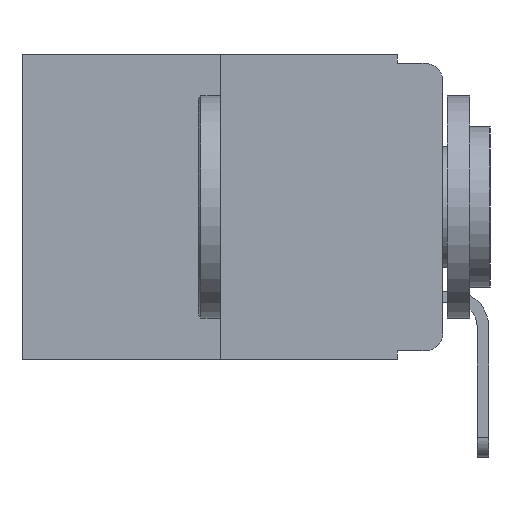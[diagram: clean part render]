
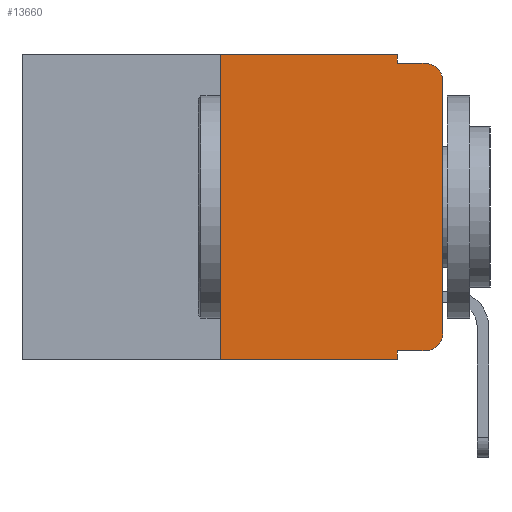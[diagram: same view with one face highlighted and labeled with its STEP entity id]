
A CAD part, left-side view. The second image highlights one B-rep face of the part: STEP entity #13660.
In plain terms, the highlighted planar face has unit normal (-1, 0, 0).
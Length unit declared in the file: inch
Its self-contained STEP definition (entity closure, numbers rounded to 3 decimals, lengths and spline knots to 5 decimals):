
#277 = CARTESIAN_POINT ( 'NONE',  ( 0., 0.473, 0. ) ) ;
#545 = CARTESIAN_POINT ( 'NONE',  ( 0., 0.051, -0.333 ) ) ;
#562 = VECTOR ( 'NONE', #14530, 39.37008 ) ;
#565 = VERTEX_POINT ( 'NONE', #15403 ) ;
#642 = ORIENTED_EDGE ( 'NONE', *, *, #10337, .F. ) ;
#785 = AXIS2_PLACEMENT_3D ( 'NONE', #16993, #5685, #18240 ) ;
#997 = EDGE_CURVE ( 'NONE', #3370, #19169, #12479, .T. ) ;
#1259 = VERTEX_POINT ( 'NONE', #2451 ) ;
#1300 = CARTESIAN_POINT ( 'NONE',  ( 0., 0.051, 0. ) ) ;
#1331 = DIRECTION ( 'NONE',  ( 0., 0., 1. ) ) ;
#1511 = LINE ( 'NONE', #11791, #12789 ) ;
#2163 = CARTESIAN_POINT ( 'NONE',  ( 0., 0.25, 0. ) ) ;
#2451 = CARTESIAN_POINT ( 'NONE',  ( 0., 0.051, -0.333 ) ) ;
#2535 = ORIENTED_EDGE ( 'NONE', *, *, #15101, .T. ) ;
#2546 = VECTOR ( 'NONE', #19663, 39.37008 ) ;
#3309 = CARTESIAN_POINT ( 'NONE',  ( 0., 0.02, -0.01 ) ) ;
#3370 = VERTEX_POINT ( 'NONE', #16117 ) ;
#3444 = DIRECTION ( 'NONE',  ( 0., 0., -1. ) ) ;
#3614 = CARTESIAN_POINT ( 'NONE',  ( 0., 0.02, -0.333 ) ) ;
#4034 = DIRECTION ( 'NONE',  ( 0., -1., 0. ) ) ;
#4049 = PLANE ( 'NONE',  #22267 ) ;
#4301 = VECTOR ( 'NONE', #3444, 39.37008 ) ;
#4721 = EDGE_CURVE ( 'NONE', #1259, #565, #16608, .T. ) ;
#5536 = CARTESIAN_POINT ( 'NONE',  ( 0., 0., -0.03 ) ) ;
#5542 = LINE ( 'NONE', #545, #12855 ) ;
#5685 = DIRECTION ( 'NONE',  ( -1., 0., 0. ) ) ;
#6744 = EDGE_CURVE ( 'NONE', #1259, #9199, #5542, .T. ) ;
#7219 = DIRECTION ( 'NONE',  ( 0., -1., 0. ) ) ;
#7855 = EDGE_LOOP ( 'NONE', ( #20491, #21220, #642, #18988, #18278, #23201, #21360, #14819, #9843, #2535 ) ) ;
#8640 = CARTESIAN_POINT ( 'NONE',  ( 0., 0., -0.313 ) ) ;
#9078 = LINE ( 'NONE', #12484, #4301 ) ;
#9199 = VERTEX_POINT ( 'NONE', #3614 ) ;
#9317 = VERTEX_POINT ( 'NONE', #8640 ) ;
#9351 = CARTESIAN_POINT ( 'NONE',  ( 0., 0.25, 0. ) ) ;
#9391 = EDGE_CURVE ( 'NONE', #3370, #565, #15246, .T. ) ;
#9843 = ORIENTED_EDGE ( 'NONE', *, *, #6744, .T. ) ;
#10128 = LINE ( 'NONE', #19658, #562 ) ;
#10290 = CARTESIAN_POINT ( 'NONE',  ( 0., 0.051, -0.01 ) ) ;
#10337 = EDGE_CURVE ( 'NONE', #12223, #21347, #23029, .T. ) ;
#10462 = VECTOR ( 'NONE', #7219, 39.37008 ) ;
#10613 = AXIS2_PLACEMENT_3D ( 'NONE', #11840, #20849, #13897 ) ;
#11493 = CIRCLE ( 'NONE', #10613, 0.02 ) ;
#11791 = CARTESIAN_POINT ( 'NONE',  ( 0., 0., 0. ) ) ;
#11800 = VERTEX_POINT ( 'NONE', #5536 ) ;
#11822 = VECTOR ( 'NONE', #16459, 39.37008 ) ;
#11840 = CARTESIAN_POINT ( 'NONE',  ( 0., 0.02, -0.03 ) ) ;
#11983 = FACE_OUTER_BOUND ( 'NONE', #7855, .T. ) ;
#12223 = VERTEX_POINT ( 'NONE', #10290 ) ;
#12479 = LINE ( 'NONE', #9351, #21134 ) ;
#12484 = CARTESIAN_POINT ( 'NONE',  ( 0., 0.051, 0. ) ) ;
#12732 = DIRECTION ( 'NONE',  ( 0., 0., 1. ) ) ;
#12789 = VECTOR ( 'NONE', #1331, 39.37008 ) ;
#12852 = DIRECTION ( 'NONE',  ( 1., 0., 0. ) ) ;
#12855 = VECTOR ( 'NONE', #4034, 39.37008 ) ;
#13660 = ADVANCED_FACE ( 'NONE', ( #11983 ), #4049, .F. ) ;
#13897 = DIRECTION ( 'NONE',  ( 0., 0., -1. ) ) ;
#14530 = DIRECTION ( 'NONE',  ( 0., -1., 0. ) ) ;
#14819 = ORIENTED_EDGE ( 'NONE', *, *, #4721, .F. ) ;
#15101 = EDGE_CURVE ( 'NONE', #9199, #9317, #19770, .T. ) ;
#15246 = LINE ( 'NONE', #16118, #10462 ) ;
#15403 = CARTESIAN_POINT ( 'NONE',  ( 0., 0.051, -0.343 ) ) ;
#15829 = EDGE_CURVE ( 'NONE', #11800, #21347, #11493, .T. ) ;
#16117 = CARTESIAN_POINT ( 'NONE',  ( 0., 0.25, -0.343 ) ) ;
#16118 = CARTESIAN_POINT ( 'NONE',  ( 0., 0.473, -0.343 ) ) ;
#16459 = DIRECTION ( 'NONE',  ( 0., 0., -1. ) ) ;
#16608 = LINE ( 'NONE', #21822, #11822 ) ;
#16993 = CARTESIAN_POINT ( 'NONE',  ( 0., 0.02, -0.313 ) ) ;
#18220 = EDGE_CURVE ( 'NONE', #9317, #11800, #1511, .T. ) ;
#18240 = DIRECTION ( 'NONE',  ( 0., 0., -1. ) ) ;
#18278 = ORIENTED_EDGE ( 'NONE', *, *, #20774, .F. ) ;
#18829 = VERTEX_POINT ( 'NONE', #1300 ) ;
#18962 = EDGE_CURVE ( 'NONE', #18829, #12223, #9078, .T. ) ;
#18988 = ORIENTED_EDGE ( 'NONE', *, *, #18962, .F. ) ;
#19169 = VERTEX_POINT ( 'NONE', #2163 ) ;
#19658 = CARTESIAN_POINT ( 'NONE',  ( 0., 0.473, 0. ) ) ;
#19663 = DIRECTION ( 'NONE',  ( 0., -1., 0. ) ) ;
#19770 = CIRCLE ( 'NONE', #785, 0.02 ) ;
#20196 = DIRECTION ( 'NONE',  ( 0., 0., -1. ) ) ;
#20491 = ORIENTED_EDGE ( 'NONE', *, *, #18220, .T. ) ;
#20774 = EDGE_CURVE ( 'NONE', #19169, #18829, #10128, .T. ) ;
#20849 = DIRECTION ( 'NONE',  ( -1., 0., 0. ) ) ;
#21134 = VECTOR ( 'NONE', #12732, 39.37008 ) ;
#21220 = ORIENTED_EDGE ( 'NONE', *, *, #15829, .T. ) ;
#21347 = VERTEX_POINT ( 'NONE', #3309 ) ;
#21360 = ORIENTED_EDGE ( 'NONE', *, *, #9391, .T. ) ;
#21396 = CARTESIAN_POINT ( 'NONE',  ( 0., 0.051, -0.01 ) ) ;
#21822 = CARTESIAN_POINT ( 'NONE',  ( 0., 0.051, 0. ) ) ;
#22267 = AXIS2_PLACEMENT_3D ( 'NONE', #277, #12852, #20196 ) ;
#23029 = LINE ( 'NONE', #21396, #2546 ) ;
#23201 = ORIENTED_EDGE ( 'NONE', *, *, #997, .F. ) ;
